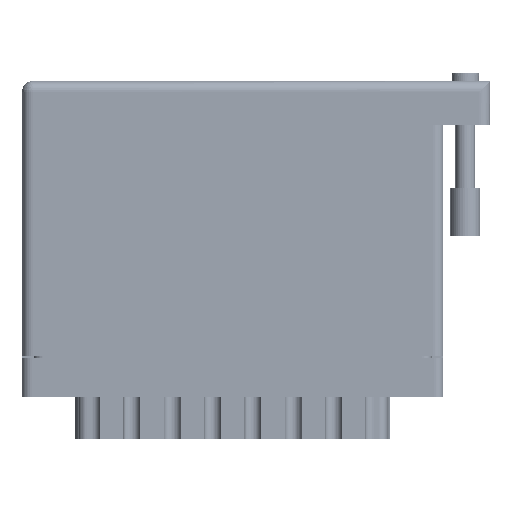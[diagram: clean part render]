
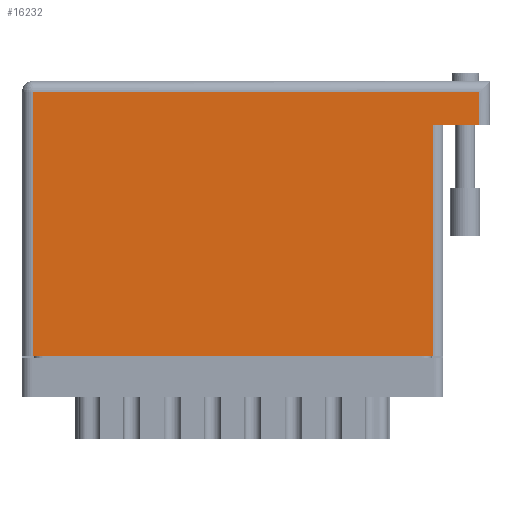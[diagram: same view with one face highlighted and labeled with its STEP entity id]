
A CAD part, front view. The second image highlights one B-rep face of the part: STEP entity #16232.
In plain terms, the highlighted face is planar.
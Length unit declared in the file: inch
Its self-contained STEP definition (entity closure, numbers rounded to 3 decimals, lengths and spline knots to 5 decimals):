
#161 = ORIENTED_EDGE ( 'NONE', *, *, #30139, .F. ) ;
#1252 = ORIENTED_EDGE ( 'NONE', *, *, #15141, .T. ) ;
#1570 = VERTEX_POINT ( 'NONE', #9027 ) ;
#3105 = VECTOR ( 'NONE', #57092, 39.37008 ) ;
#5332 = ORIENTED_EDGE ( 'NONE', *, *, #70134, .T. ) ;
#5953 = DIRECTION ( 'NONE',  ( 0., 1., 0. ) ) ;
#5979 = CARTESIAN_POINT ( 'NONE',  ( 2.948, 1.705, 0. ) ) ;
#7438 = VERTEX_POINT ( 'NONE', #60469 ) ;
#8237 = VECTOR ( 'NONE', #5953, 39.37008 ) ;
#8453 = EDGE_CURVE ( 'NONE', #41084, #66046, #51512, .T. ) ;
#9027 = CARTESIAN_POINT ( 'NONE',  ( 2.648, 0., 0. ) ) ;
#11383 = CARTESIAN_POINT ( 'NONE',  ( 2.948, 1.495, 0. ) ) ;
#13352 = VECTOR ( 'NONE', #35483, 39.37008 ) ;
#15141 = EDGE_CURVE ( 'NONE', #1570, #18373, #64982, .T. ) ;
#16232 = ADVANCED_FACE ( 'NONE', ( #58319 ), #35529, .F. ) ;
#18051 = LINE ( 'NONE', #60319, #46520 ) ;
#18373 = VERTEX_POINT ( 'NONE', #75862 ) ;
#18418 = CARTESIAN_POINT ( 'NONE',  ( 0., 1.705, 0. ) ) ;
#18584 = DIRECTION ( 'NONE',  ( -1., 0., 0. ) ) ;
#19221 = ORIENTED_EDGE ( 'NONE', *, *, #62067, .T. ) ;
#20316 = CARTESIAN_POINT ( 'NONE',  ( 0.07, 1.705, 0. ) ) ;
#22899 = VERTEX_POINT ( 'NONE', #11383 ) ;
#23446 = CARTESIAN_POINT ( 'NONE',  ( 2.648, 1.495, 0. ) ) ;
#25389 = DIRECTION ( 'NONE',  ( 0., -1., 0. ) ) ;
#29915 = CARTESIAN_POINT ( 'NONE',  ( 0., 1.775, 0. ) ) ;
#30139 = EDGE_CURVE ( 'NONE', #22899, #18373, #64752, .T. ) ;
#31526 = VECTOR ( 'NONE', #64081, 39.37008 ) ;
#35483 = DIRECTION ( 'NONE',  ( 0., 1., 0. ) ) ;
#35529 = PLANE ( 'NONE',  #40236 ) ;
#35866 = VECTOR ( 'NONE', #46707, 39.37008 ) ;
#39709 = ORIENTED_EDGE ( 'NONE', *, *, #8453, .T. ) ;
#40236 = AXIS2_PLACEMENT_3D ( 'NONE', #29915, #47889, #18584 ) ;
#41084 = VERTEX_POINT ( 'NONE', #5979 ) ;
#41193 = CARTESIAN_POINT ( 'NONE',  ( 2.948, 1.775, 0. ) ) ;
#46520 = VECTOR ( 'NONE', #25389, 39.37008 ) ;
#46707 = DIRECTION ( 'NONE',  ( -1., 0., 0. ) ) ;
#47889 = DIRECTION ( 'NONE',  ( 0., 0., -1. ) ) ;
#51512 = LINE ( 'NONE', #18418, #35866 ) ;
#51714 = LINE ( 'NONE', #70010, #31526 ) ;
#57092 = DIRECTION ( 'NONE',  ( -1., 0., 0. ) ) ;
#58319 = FACE_OUTER_BOUND ( 'NONE', #74131, .T. ) ;
#60319 = CARTESIAN_POINT ( 'NONE',  ( 0.07, 0., 0. ) ) ;
#60469 = CARTESIAN_POINT ( 'NONE',  ( 0.07, 0., 0. ) ) ;
#62067 = EDGE_CURVE ( 'NONE', #7438, #1570, #51714, .T. ) ;
#62783 = CARTESIAN_POINT ( 'NONE',  ( 3.018, 1.495, 0. ) ) ;
#62817 = ORIENTED_EDGE ( 'NONE', *, *, #66608, .T. ) ;
#64081 = DIRECTION ( 'NONE',  ( 1., 0., 0. ) ) ;
#64752 = LINE ( 'NONE', #62783, #3105 ) ;
#64982 = LINE ( 'NONE', #23446, #13352 ) ;
#66046 = VERTEX_POINT ( 'NONE', #20316 ) ;
#66608 = EDGE_CURVE ( 'NONE', #66046, #7438, #18051, .T. ) ;
#70010 = CARTESIAN_POINT ( 'NONE',  ( 0., 0., 0. ) ) ;
#70134 = EDGE_CURVE ( 'NONE', #22899, #41084, #71796, .T. ) ;
#71796 = LINE ( 'NONE', #41193, #8237 ) ;
#74131 = EDGE_LOOP ( 'NONE', ( #19221, #1252, #161, #5332, #39709, #62817 ) ) ;
#75862 = CARTESIAN_POINT ( 'NONE',  ( 2.648, 1.495, 0. ) ) ;
